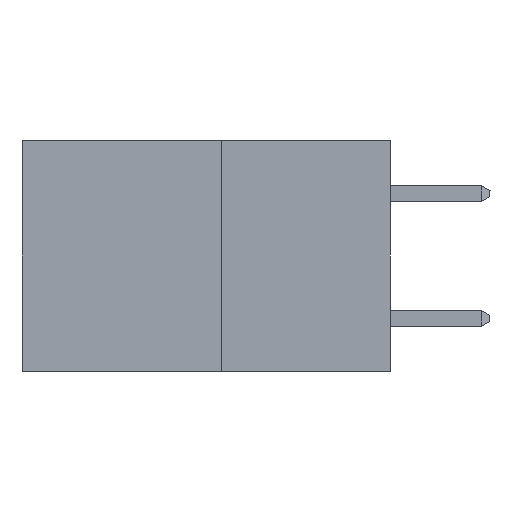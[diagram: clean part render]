
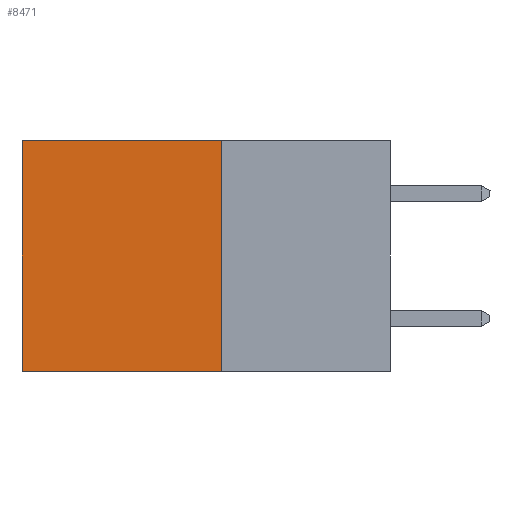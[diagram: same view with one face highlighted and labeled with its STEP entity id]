
A CAD part, left-side view. The second image highlights one B-rep face of the part: STEP entity #8471.
In plain terms, the highlighted planar face has unit normal (-1, 0, 0).
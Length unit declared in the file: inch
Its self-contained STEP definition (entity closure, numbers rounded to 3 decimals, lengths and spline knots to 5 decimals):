
#1154 = CARTESIAN_POINT ( 'NONE',  ( 0.277, 0.27, -0.37 ) ) ;
#1283 = VECTOR ( 'NONE', #3375, 39.37008 ) ;
#1742 = CARTESIAN_POINT ( 'NONE',  ( 0.277, 0.27, -0.37 ) ) ;
#2168 = DIRECTION ( 'NONE',  ( 0., 0., -1. ) ) ;
#2266 = DIRECTION ( 'NONE',  ( 0., 1., 0. ) ) ;
#2362 = CARTESIAN_POINT ( 'NONE',  ( 0.277, 0.27, 0. ) ) ;
#2384 = CARTESIAN_POINT ( 'NONE',  ( 0.277, 0.59, -0.37 ) ) ;
#2504 = LINE ( 'NONE', #2545, #7724 ) ;
#2545 = CARTESIAN_POINT ( 'NONE',  ( 0.277, 0.27, -0.37 ) ) ;
#3045 = ORIENTED_EDGE ( 'NONE', *, *, #3554, .T. ) ;
#3375 = DIRECTION ( 'NONE',  ( 0., 0., -1. ) ) ;
#3554 = EDGE_CURVE ( 'NONE', #5358, #10320, #12012, .T. ) ;
#4200 = AXIS2_PLACEMENT_3D ( 'NONE', #1154, #8024, #2168 ) ;
#4221 = LINE ( 'NONE', #2384, #1283 ) ;
#4695 = EDGE_CURVE ( 'NONE', #10320, #11256, #4221, .T. ) ;
#4732 = ORIENTED_EDGE ( 'NONE', *, *, #9270, .F. ) ;
#4885 = ORIENTED_EDGE ( 'NONE', *, *, #4695, .T. ) ;
#4950 = VERTEX_POINT ( 'NONE', #1742 ) ;
#5358 = VERTEX_POINT ( 'NONE', #2362 ) ;
#5652 = ORIENTED_EDGE ( 'NONE', *, *, #11681, .F. ) ;
#6042 = FACE_OUTER_BOUND ( 'NONE', #11160, .T. ) ;
#6126 = CARTESIAN_POINT ( 'NONE',  ( 0.277, 0.59, 0. ) ) ;
#6133 = LINE ( 'NONE', #9107, #9013 ) ;
#7650 = CARTESIAN_POINT ( 'NONE',  ( 0.277, 0.27, 0. ) ) ;
#7724 = VECTOR ( 'NONE', #9368, 39.37008 ) ;
#8024 = DIRECTION ( 'NONE',  ( 1., 0., 0. ) ) ;
#8471 = ADVANCED_FACE ( 'NONE', ( #6042 ), #10941, .F. ) ;
#8612 = DIRECTION ( 'NONE',  ( 0., 1., 0. ) ) ;
#9013 = VECTOR ( 'NONE', #2266, 39.37008 ) ;
#9107 = CARTESIAN_POINT ( 'NONE',  ( 0.277, 0.27, -0.37 ) ) ;
#9270 = EDGE_CURVE ( 'NONE', #5358, #4950, #2504, .T. ) ;
#9368 = DIRECTION ( 'NONE',  ( 0., 0., -1. ) ) ;
#9453 = CARTESIAN_POINT ( 'NONE',  ( 0.277, 0.59, -0.37 ) ) ;
#10320 = VERTEX_POINT ( 'NONE', #6126 ) ;
#10941 = PLANE ( 'NONE',  #4200 ) ;
#11160 = EDGE_LOOP ( 'NONE', ( #4885, #5652, #4732, #3045 ) ) ;
#11256 = VERTEX_POINT ( 'NONE', #9453 ) ;
#11575 = VECTOR ( 'NONE', #8612, 39.37008 ) ;
#11681 = EDGE_CURVE ( 'NONE', #4950, #11256, #6133, .T. ) ;
#12012 = LINE ( 'NONE', #7650, #11575 ) ;
